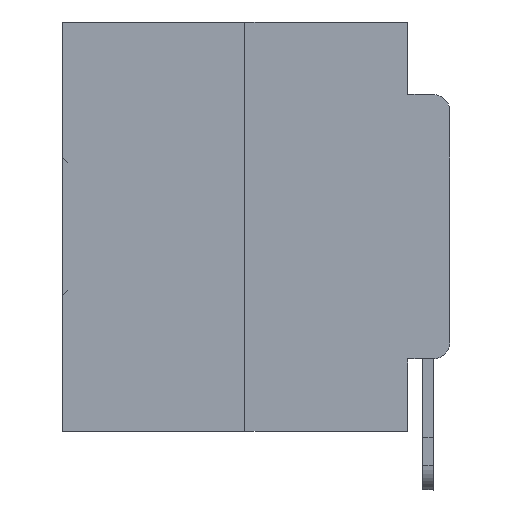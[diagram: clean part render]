
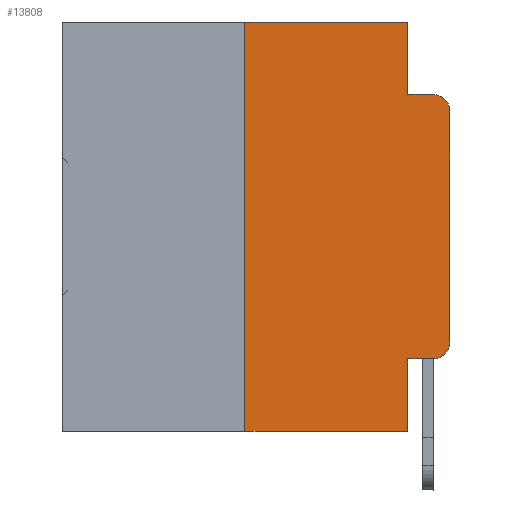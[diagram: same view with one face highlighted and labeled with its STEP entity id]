
A CAD part, left-side view. The second image highlights one B-rep face of the part: STEP entity #13808.
In plain terms, the highlighted planar face has unit normal (-1, 0, 0).
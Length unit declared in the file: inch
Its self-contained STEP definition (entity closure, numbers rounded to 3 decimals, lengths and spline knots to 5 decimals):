
#250 = CIRCLE ( 'NONE', #1098, 0.02 ) ;
#373 = VECTOR ( 'NONE', #18090, 39.37008 ) ;
#417 = LINE ( 'NONE', #16653, #14721 ) ;
#835 = ORIENTED_EDGE ( 'NONE', *, *, #29698, .T. ) ;
#1085 = LINE ( 'NONE', #27857, #11073 ) ;
#1098 = AXIS2_PLACEMENT_3D ( 'NONE', #7383, #20865, #26274 ) ;
#1115 = ORIENTED_EDGE ( 'NONE', *, *, #16829, .T. ) ;
#1881 = DIRECTION ( 'NONE',  ( 1., 0., 0. ) ) ;
#3166 = CARTESIAN_POINT ( 'NONE',  ( 0., 0., -0.3915 ) ) ;
#3765 = LINE ( 'NONE', #15913, #15542 ) ;
#3926 = DIRECTION ( 'NONE',  ( 0., -1., 0. ) ) ;
#4188 = CARTESIAN_POINT ( 'NONE',  ( 0., 0.25, 0. ) ) ;
#4583 = ORIENTED_EDGE ( 'NONE', *, *, #33822, .F. ) ;
#4790 = DIRECTION ( 'NONE',  ( 0., -1., 0. ) ) ;
#5042 = CARTESIAN_POINT ( 'NONE',  ( 0., 0.051, -0.5 ) ) ;
#6213 = CARTESIAN_POINT ( 'NONE',  ( 0., 0.051, -0.4115 ) ) ;
#6764 = LINE ( 'NONE', #22893, #19305 ) ;
#6940 = VERTEX_POINT ( 'NONE', #21070 ) ;
#7092 = CARTESIAN_POINT ( 'NONE',  ( 0., 0.051, 0. ) ) ;
#7289 = EDGE_CURVE ( 'NONE', #33485, #24638, #6764, .T. ) ;
#7383 = CARTESIAN_POINT ( 'NONE',  ( 0., 0.02, -0.1085 ) ) ;
#8179 = EDGE_CURVE ( 'NONE', #17593, #26071, #18444, .T. ) ;
#8407 = VECTOR ( 'NONE', #32931, 39.37008 ) ;
#8499 = EDGE_CURVE ( 'NONE', #12264, #6940, #8696, .T. ) ;
#8696 = LINE ( 'NONE', #17971, #373 ) ;
#9034 = EDGE_CURVE ( 'NONE', #26761, #24638, #1085, .T. ) ;
#9524 = CARTESIAN_POINT ( 'NONE',  ( 0., 0.02, -0.3915 ) ) ;
#9752 = ORIENTED_EDGE ( 'NONE', *, *, #8499, .F. ) ;
#11028 = VECTOR ( 'NONE', #17101, 39.37008 ) ;
#11073 = VECTOR ( 'NONE', #3926, 39.37008 ) ;
#11443 = CARTESIAN_POINT ( 'NONE',  ( 0., 0.051, -0.4115 ) ) ;
#11545 = VERTEX_POINT ( 'NONE', #30136 ) ;
#11961 = ORIENTED_EDGE ( 'NONE', *, *, #23192, .F. ) ;
#11993 = CARTESIAN_POINT ( 'NONE',  ( 0., 0., -0.1085 ) ) ;
#12252 = DIRECTION ( 'NONE',  ( 0., 0., -1. ) ) ;
#12264 = VERTEX_POINT ( 'NONE', #7092 ) ;
#12493 = DIRECTION ( 'NONE',  ( 0., 0., 1. ) ) ;
#12955 = DIRECTION ( 'NONE',  ( 0., 0., 1. ) ) ;
#13808 = ADVANCED_FACE ( 'NONE', ( #14124 ), #15098, .F. ) ;
#14124 = FACE_OUTER_BOUND ( 'NONE', #28185, .T. ) ;
#14721 = VECTOR ( 'NONE', #12493, 39.37008 ) ;
#15098 = PLANE ( 'NONE',  #25638 ) ;
#15542 = VECTOR ( 'NONE', #4790, 39.37008 ) ;
#15913 = CARTESIAN_POINT ( 'NONE',  ( 0., 0.051, -0.0885 ) ) ;
#16653 = CARTESIAN_POINT ( 'NONE',  ( 0., 0.25, 0. ) ) ;
#16829 = EDGE_CURVE ( 'NONE', #29157, #11545, #250, .T. ) ;
#17101 = DIRECTION ( 'NONE',  ( 0., -1., 0. ) ) ;
#17593 = VERTEX_POINT ( 'NONE', #25818 ) ;
#17971 = CARTESIAN_POINT ( 'NONE',  ( 0., 0.051, 0. ) ) ;
#18090 = DIRECTION ( 'NONE',  ( 0., 0., -1. ) ) ;
#18183 = LINE ( 'NONE', #6213, #11028 ) ;
#18263 = EDGE_CURVE ( 'NONE', #33485, #17593, #18183, .T. ) ;
#18327 = ORIENTED_EDGE ( 'NONE', *, *, #9034, .T. ) ;
#18444 = CIRCLE ( 'NONE', #25272, 0.02 ) ;
#18924 = LINE ( 'NONE', #25084, #8407 ) ;
#19305 = VECTOR ( 'NONE', #26175, 39.37008 ) ;
#20034 = EDGE_CURVE ( 'NONE', #26761, #27587, #417, .T. ) ;
#20590 = DIRECTION ( 'NONE',  ( 0., 0., -1. ) ) ;
#20845 = ORIENTED_EDGE ( 'NONE', *, *, #18263, .T. ) ;
#20865 = DIRECTION ( 'NONE',  ( -1., 0., 0. ) ) ;
#21070 = CARTESIAN_POINT ( 'NONE',  ( 0., 0.051, -0.0885 ) ) ;
#22893 = CARTESIAN_POINT ( 'NONE',  ( 0., 0.051, 0. ) ) ;
#23192 = EDGE_CURVE ( 'NONE', #27587, #12264, #18924, .T. ) ;
#23409 = ORIENTED_EDGE ( 'NONE', *, *, #7289, .F. ) ;
#24638 = VERTEX_POINT ( 'NONE', #5042 ) ;
#25084 = CARTESIAN_POINT ( 'NONE',  ( 0., 0.473, 0. ) ) ;
#25272 = AXIS2_PLACEMENT_3D ( 'NONE', #9524, #28213, #12252 ) ;
#25638 = AXIS2_PLACEMENT_3D ( 'NONE', #26135, #1881, #20590 ) ;
#25818 = CARTESIAN_POINT ( 'NONE',  ( 0., 0.02, -0.4115 ) ) ;
#26071 = VERTEX_POINT ( 'NONE', #3166 ) ;
#26135 = CARTESIAN_POINT ( 'NONE',  ( 0., 0.473, 0. ) ) ;
#26175 = DIRECTION ( 'NONE',  ( 0., 0., -1. ) ) ;
#26274 = DIRECTION ( 'NONE',  ( 0., 0., -1. ) ) ;
#26328 = CARTESIAN_POINT ( 'NONE',  ( 0., 0., 0. ) ) ;
#26746 = ORIENTED_EDGE ( 'NONE', *, *, #8179, .T. ) ;
#26761 = VERTEX_POINT ( 'NONE', #32160 ) ;
#27302 = VECTOR ( 'NONE', #12955, 39.37008 ) ;
#27587 = VERTEX_POINT ( 'NONE', #4188 ) ;
#27857 = CARTESIAN_POINT ( 'NONE',  ( 0., 0.473, -0.5 ) ) ;
#28185 = EDGE_LOOP ( 'NONE', ( #835, #1115, #4583, #9752, #11961, #28289, #18327, #23409, #20845, #26746 ) ) ;
#28213 = DIRECTION ( 'NONE',  ( -1., 0., 0. ) ) ;
#28289 = ORIENTED_EDGE ( 'NONE', *, *, #20034, .F. ) ;
#29157 = VERTEX_POINT ( 'NONE', #11993 ) ;
#29698 = EDGE_CURVE ( 'NONE', #26071, #29157, #34352, .T. ) ;
#30136 = CARTESIAN_POINT ( 'NONE',  ( 0., 0.02, -0.0885 ) ) ;
#32160 = CARTESIAN_POINT ( 'NONE',  ( 0., 0.25, -0.5 ) ) ;
#32931 = DIRECTION ( 'NONE',  ( 0., -1., 0. ) ) ;
#33485 = VERTEX_POINT ( 'NONE', #11443 ) ;
#33822 = EDGE_CURVE ( 'NONE', #6940, #11545, #3765, .T. ) ;
#34352 = LINE ( 'NONE', #26328, #27302 ) ;
